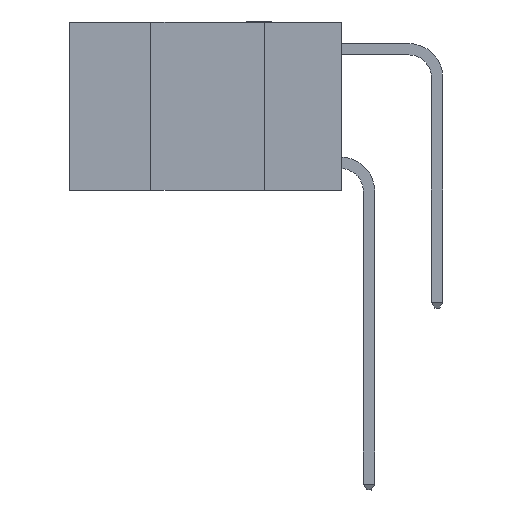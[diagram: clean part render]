
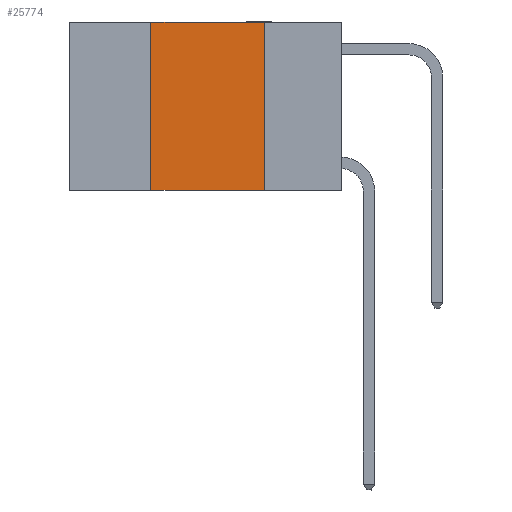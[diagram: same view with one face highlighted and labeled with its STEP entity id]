
A CAD part, left-side view. The second image highlights one B-rep face of the part: STEP entity #25774.
In plain terms, the highlighted planar face has unit normal (-1, 0, 0).
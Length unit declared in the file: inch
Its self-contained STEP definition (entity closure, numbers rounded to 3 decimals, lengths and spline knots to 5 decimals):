
#340 = CARTESIAN_POINT ( 'NONE',  ( 0., 0.6, 0. ) ) ;
#583 = VERTEX_POINT ( 'NONE', #10361 ) ;
#928 = LINE ( 'NONE', #6873, #19436 ) ;
#1727 = VECTOR ( 'NONE', #6497, 39.37008 ) ;
#2556 = AXIS2_PLACEMENT_3D ( 'NONE', #340, #20847, #22712 ) ;
#2665 = LINE ( 'NONE', #22916, #1727 ) ;
#3754 = CARTESIAN_POINT ( 'NONE',  ( 0., 0.42, 0. ) ) ;
#4368 = DIRECTION ( 'NONE',  ( 0., -1., 0. ) ) ;
#5162 = VERTEX_POINT ( 'NONE', #7136 ) ;
#5192 = DIRECTION ( 'NONE',  ( 0., 0., -1. ) ) ;
#5959 = VERTEX_POINT ( 'NONE', #12514 ) ;
#6197 = EDGE_CURVE ( 'NONE', #5959, #5162, #2665, .T. ) ;
#6497 = DIRECTION ( 'NONE',  ( 0., -1., 0. ) ) ;
#6653 = VECTOR ( 'NONE', #18880, 39.37008 ) ;
#6873 = CARTESIAN_POINT ( 'NONE',  ( 0., 0.6, 0. ) ) ;
#7136 = CARTESIAN_POINT ( 'NONE',  ( 0., 0.17, -0.37 ) ) ;
#8103 = EDGE_LOOP ( 'NONE', ( #18772, #14491, #20044, #19514 ) ) ;
#8521 = EDGE_CURVE ( 'NONE', #583, #5162, #23325, .T. ) ;
#10361 = CARTESIAN_POINT ( 'NONE',  ( 0., 0.17, 0. ) ) ;
#11153 = CARTESIAN_POINT ( 'NONE',  ( 0., 0.17, 0. ) ) ;
#12514 = CARTESIAN_POINT ( 'NONE',  ( 0., 0.42, -0.37 ) ) ;
#14491 = ORIENTED_EDGE ( 'NONE', *, *, #23717, .F. ) ;
#14749 = PLANE ( 'NONE',  #2556 ) ;
#14895 = LINE ( 'NONE', #22984, #6653 ) ;
#16610 = FACE_OUTER_BOUND ( 'NONE', #8103, .T. ) ;
#18772 = ORIENTED_EDGE ( 'NONE', *, *, #8521, .F. ) ;
#18880 = DIRECTION ( 'NONE',  ( 0., 0., 1. ) ) ;
#19436 = VECTOR ( 'NONE', #4368, 39.37008 ) ;
#19514 = ORIENTED_EDGE ( 'NONE', *, *, #6197, .T. ) ;
#20044 = ORIENTED_EDGE ( 'NONE', *, *, #20485, .F. ) ;
#20485 = EDGE_CURVE ( 'NONE', #5959, #26054, #14895, .T. ) ;
#20847 = DIRECTION ( 'NONE',  ( 1., 0., 0. ) ) ;
#22712 = DIRECTION ( 'NONE',  ( 0., 0., -1. ) ) ;
#22916 = CARTESIAN_POINT ( 'NONE',  ( 0., 0.6, -0.37 ) ) ;
#22984 = CARTESIAN_POINT ( 'NONE',  ( 0., 0.42, 0. ) ) ;
#23308 = VECTOR ( 'NONE', #5192, 39.37008 ) ;
#23325 = LINE ( 'NONE', #11153, #23308 ) ;
#23717 = EDGE_CURVE ( 'NONE', #26054, #583, #928, .T. ) ;
#25774 = ADVANCED_FACE ( 'NONE', ( #16610 ), #14749, .F. ) ;
#26054 = VERTEX_POINT ( 'NONE', #3754 ) ;
